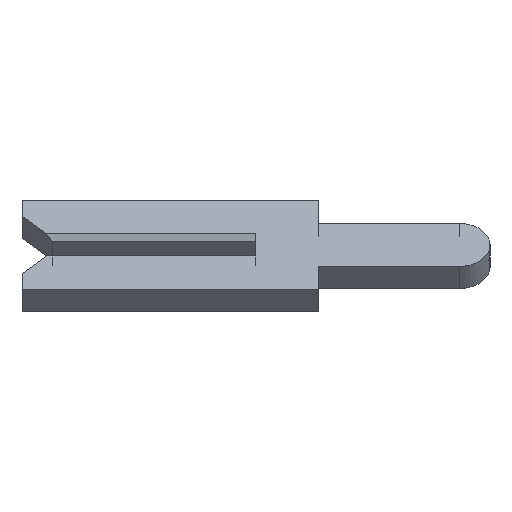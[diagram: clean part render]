
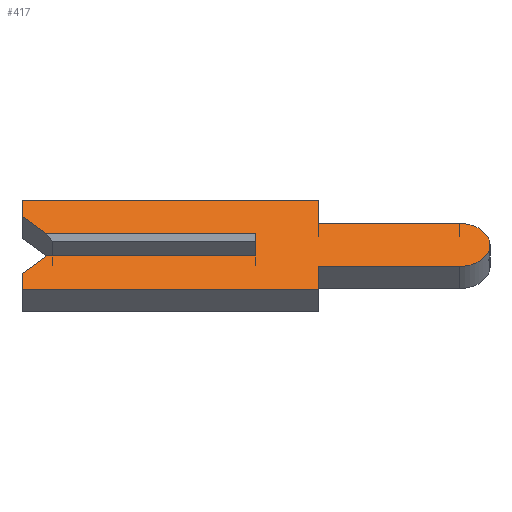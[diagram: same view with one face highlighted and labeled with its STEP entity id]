
A CAD part, left-side view. The second image highlights one B-rep face of the part: STEP entity #417.
In plain terms, the highlighted face is planar.
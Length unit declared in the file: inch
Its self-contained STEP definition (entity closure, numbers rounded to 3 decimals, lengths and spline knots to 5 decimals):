
#7 = ORIENTED_EDGE ( 'NONE', *, *, #1251, .F. ) ;
#15 = CARTESIAN_POINT ( 'NONE',  ( -0.01, -0.04, 0.04 ) ) ;
#16 = VERTEX_POINT ( 'NONE', #1061 ) ;
#64 = DIRECTION ( 'NONE',  ( 0., 0., -1. ) ) ;
#77 = VERTEX_POINT ( 'NONE', #15 ) ;
#107 = FACE_OUTER_BOUND ( 'NONE', #122, .T. ) ;
#108 = DIRECTION ( 'NONE',  ( 0., -1., 0. ) ) ;
#122 = EDGE_LOOP ( 'NONE', ( #1775, #2048, #892, #1806, #1841, #1241, #693, #7, #545, #1876, #340, #371, #569, #646 ) ) ;
#158 = VECTOR ( 'NONE', #752, 39.37008 ) ;
#195 = VECTOR ( 'NONE', #1028, 39.37008 ) ;
#210 = CARTESIAN_POINT ( 'NONE',  ( -0.01, 0.15, -0.04 ) ) ;
#219 = LINE ( 'NONE', #1925, #195 ) ;
#242 = CARTESIAN_POINT ( 'NONE',  ( -0.01, -0.1305, 0. ) ) ;
#249 = EDGE_CURVE ( 'NONE', #2099, #1045, #1970, .T. ) ;
#265 = LINE ( 'NONE', #959, #1358 ) ;
#278 = CARTESIAN_POINT ( 'NONE',  ( -0.01, -0.04, -0.0195 ) ) ;
#326 = CARTESIAN_POINT ( 'NONE',  ( -0.01, 0.1305, 0.0065 ) ) ;
#334 = CARTESIAN_POINT ( 'NONE',  ( -0.01, -0.04, -0.04 ) ) ;
#340 = ORIENTED_EDGE ( 'NONE', *, *, #1507, .F. ) ;
#352 = VECTOR ( 'NONE', #744, 39.37008 ) ;
#371 = ORIENTED_EDGE ( 'NONE', *, *, #1104, .F. ) ;
#379 = LINE ( 'NONE', #2180, #1726 ) ;
#417 = ADVANCED_FACE ( 'NONE', ( #107 ), #572, .F. ) ;
#485 = CARTESIAN_POINT ( 'NONE',  ( -0.01, 0.15, 0.04 ) ) ;
#497 = AXIS2_PLACEMENT_3D ( 'NONE', #242, #2155, #926 ) ;
#521 = DIRECTION ( 'NONE',  ( 0., 0., -1. ) ) ;
#545 = ORIENTED_EDGE ( 'NONE', *, *, #703, .F. ) ;
#558 = VERTEX_POINT ( 'NONE', #1965 ) ;
#569 = ORIENTED_EDGE ( 'NONE', *, *, #918, .F. ) ;
#572 = PLANE ( 'NONE',  #497 ) ;
#641 = CARTESIAN_POINT ( 'NONE',  ( -0.01, 0.134, -0.01 ) ) ;
#646 = ORIENTED_EDGE ( 'NONE', *, *, #2023, .F. ) ;
#654 = DIRECTION ( 'NONE',  ( 0., 0., 1. ) ) ;
#676 = EDGE_CURVE ( 'NONE', #16, #1327, #1445, .T. ) ;
#688 = LINE ( 'NONE', #788, #1252 ) ;
#693 = ORIENTED_EDGE ( 'NONE', *, *, #2036, .F. ) ;
#695 = VERTEX_POINT ( 'NONE', #914 ) ;
#703 = EDGE_CURVE ( 'NONE', #2157, #558, #1884, .T. ) ;
#723 = VECTOR ( 'NONE', #1564, 39.37008 ) ;
#744 = DIRECTION ( 'NONE',  ( 0., -0.707, 0.707 ) ) ;
#752 = DIRECTION ( 'NONE',  ( 0., 1., 0. ) ) ;
#788 = CARTESIAN_POINT ( 'NONE',  ( -0.01, 0.15, 0.01 ) ) ;
#833 = DIRECTION ( 'NONE',  ( 0., 0., -1. ) ) ;
#892 = ORIENTED_EDGE ( 'NONE', *, *, #2226, .F. ) ;
#914 = CARTESIAN_POINT ( 'NONE',  ( -0.01, 0., -0.01 ) ) ;
#918 = EDGE_CURVE ( 'NONE', #1151, #1463, #1910, .T. ) ;
#926 = DIRECTION ( 'NONE',  ( 0., 0., -1. ) ) ;
#959 = CARTESIAN_POINT ( 'NONE',  ( -0.01, 0.15, 0.04 ) ) ;
#967 = CARTESIAN_POINT ( 'NONE',  ( -0.01, 0., 0.01 ) ) ;
#991 = CARTESIAN_POINT ( 'NONE',  ( -0.01, 0.134, 0.01 ) ) ;
#997 = EDGE_CURVE ( 'NONE', #1433, #1085, #688, .T. ) ;
#1019 = VERTEX_POINT ( 'NONE', #278 ) ;
#1028 = DIRECTION ( 'NONE',  ( 0., -1., 0. ) ) ;
#1045 = VERTEX_POINT ( 'NONE', #641 ) ;
#1046 = CARTESIAN_POINT ( 'NONE',  ( -0.01, -0.1305, 0.0195 ) ) ;
#1061 = CARTESIAN_POINT ( 'NONE',  ( -0.01, -0.04, -0.04 ) ) ;
#1085 = VERTEX_POINT ( 'NONE', #967 ) ;
#1087 = DIRECTION ( 'NONE',  ( 1., 0., 0. ) ) ;
#1104 = EDGE_CURVE ( 'NONE', #1463, #77, #265, .T. ) ;
#1139 = CARTESIAN_POINT ( 'NONE',  ( -0.01, 0.15, 0.026 ) ) ;
#1151 = VERTEX_POINT ( 'NONE', #1478 ) ;
#1179 = VECTOR ( 'NONE', #521, 39.37008 ) ;
#1207 = CARTESIAN_POINT ( 'NONE',  ( -0.01, 0.15, -0.026 ) ) ;
#1228 = CARTESIAN_POINT ( 'NONE',  ( -0.01, 0.15, -0.026 ) ) ;
#1241 = ORIENTED_EDGE ( 'NONE', *, *, #676, .F. ) ;
#1251 = EDGE_CURVE ( 'NONE', #558, #1019, #379, .T. ) ;
#1252 = VECTOR ( 'NONE', #2005, 39.37008 ) ;
#1262 = VERTEX_POINT ( 'NONE', #2016 ) ;
#1268 = LINE ( 'NONE', #334, #1179 ) ;
#1315 = DIRECTION ( 'NONE',  ( 0., 0., 1. ) ) ;
#1327 = VERTEX_POINT ( 'NONE', #2222 ) ;
#1358 = VECTOR ( 'NONE', #108, 39.37008 ) ;
#1422 = DIRECTION ( 'NONE',  ( 0., -1., 0. ) ) ;
#1433 = VERTEX_POINT ( 'NONE', #991 ) ;
#1445 = LINE ( 'NONE', #210, #158 ) ;
#1463 = VERTEX_POINT ( 'NONE', #485 ) ;
#1478 = CARTESIAN_POINT ( 'NONE',  ( -0.01, 0.15, 0.026 ) ) ;
#1507 = EDGE_CURVE ( 'NONE', #77, #1262, #2203, .T. ) ;
#1562 = VECTOR ( 'NONE', #1422, 39.37008 ) ;
#1564 = DIRECTION ( 'NONE',  ( 0., 0., 1. ) ) ;
#1581 = EDGE_CURVE ( 'NONE', #695, #1085, #2136, .T. ) ;
#1652 = VECTOR ( 'NONE', #1908, 39.37008 ) ;
#1664 = VECTOR ( 'NONE', #1315, 39.37008 ) ;
#1696 = CARTESIAN_POINT ( 'NONE',  ( -0.01, 0., 0.0065 ) ) ;
#1702 = CARTESIAN_POINT ( 'NONE',  ( -0.01, -0.04, 0.04 ) ) ;
#1726 = VECTOR ( 'NONE', #2024, 39.37008 ) ;
#1775 = ORIENTED_EDGE ( 'NONE', *, *, #997, .T. ) ;
#1806 = ORIENTED_EDGE ( 'NONE', *, *, #249, .F. ) ;
#1811 = CARTESIAN_POINT ( 'NONE',  ( -0.01, -0.1305, 0. ) ) ;
#1841 = ORIENTED_EDGE ( 'NONE', *, *, #2147, .F. ) ;
#1876 = ORIENTED_EDGE ( 'NONE', *, *, #2162, .F. ) ;
#1884 = CIRCLE ( 'NONE', #2137, 0.0195 ) ;
#1908 = DIRECTION ( 'NONE',  ( 0., 0.707, 0.707 ) ) ;
#1910 = LINE ( 'NONE', #1139, #1664 ) ;
#1925 = CARTESIAN_POINT ( 'NONE',  ( -0.01, -0.04, 0.0195 ) ) ;
#1965 = CARTESIAN_POINT ( 'NONE',  ( -0.01, -0.1305, -0.0195 ) ) ;
#1970 = LINE ( 'NONE', #1988, #352 ) ;
#1975 = VECTOR ( 'NONE', #654, 39.37008 ) ;
#1988 = CARTESIAN_POINT ( 'NONE',  ( -0.01, 0.1305, -0.0065 ) ) ;
#2002 = VECTOR ( 'NONE', #833, 39.37008 ) ;
#2005 = DIRECTION ( 'NONE',  ( 0., -1., 0. ) ) ;
#2015 = LINE ( 'NONE', #326, #1652 ) ;
#2016 = CARTESIAN_POINT ( 'NONE',  ( -0.01, -0.04, 0.0195 ) ) ;
#2023 = EDGE_CURVE ( 'NONE', #1433, #1151, #2015, .T. ) ;
#2024 = DIRECTION ( 'NONE',  ( 0., 1., 0. ) ) ;
#2036 = EDGE_CURVE ( 'NONE', #1019, #16, #1268, .T. ) ;
#2048 = ORIENTED_EDGE ( 'NONE', *, *, #1581, .F. ) ;
#2071 = LINE ( 'NONE', #2139, #1562 ) ;
#2099 = VERTEX_POINT ( 'NONE', #1207 ) ;
#2136 = LINE ( 'NONE', #1696, #1975 ) ;
#2137 = AXIS2_PLACEMENT_3D ( 'NONE', #1811, #1087, #64 ) ;
#2139 = CARTESIAN_POINT ( 'NONE',  ( -0.01, -0.1305, -0.01 ) ) ;
#2147 = EDGE_CURVE ( 'NONE', #1327, #2099, #2173, .T. ) ;
#2155 = DIRECTION ( 'NONE',  ( 1., 0., 0. ) ) ;
#2157 = VERTEX_POINT ( 'NONE', #1046 ) ;
#2162 = EDGE_CURVE ( 'NONE', #1262, #2157, #219, .T. ) ;
#2173 = LINE ( 'NONE', #1228, #723 ) ;
#2180 = CARTESIAN_POINT ( 'NONE',  ( -0.01, -0.04, -0.0195 ) ) ;
#2203 = LINE ( 'NONE', #1702, #2002 ) ;
#2222 = CARTESIAN_POINT ( 'NONE',  ( -0.01, 0.15, -0.04 ) ) ;
#2226 = EDGE_CURVE ( 'NONE', #1045, #695, #2071, .T. ) ;
